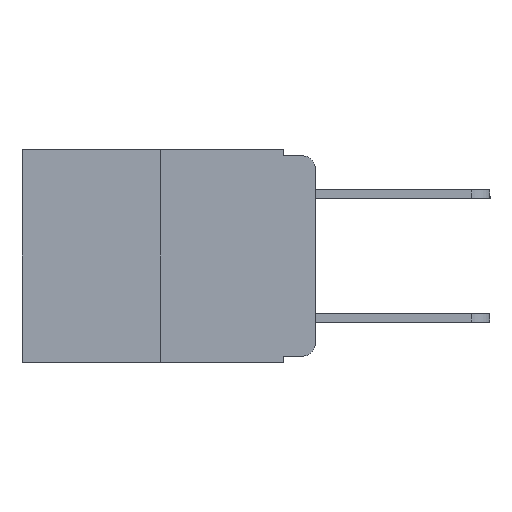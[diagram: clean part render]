
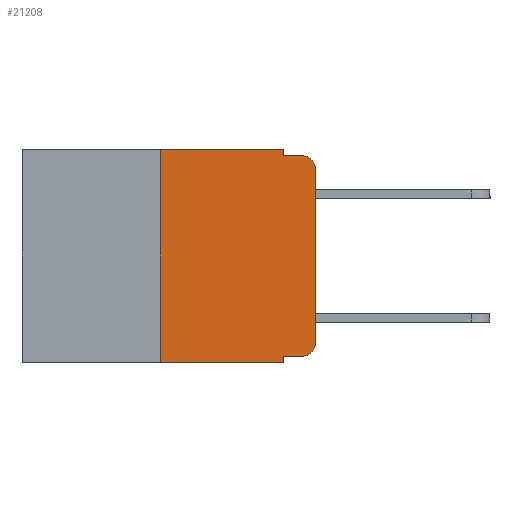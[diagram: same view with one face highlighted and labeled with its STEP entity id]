
A CAD part, left-side view. The second image highlights one B-rep face of the part: STEP entity #21208.
In plain terms, the highlighted planar face has unit normal (-1, 0, 0).
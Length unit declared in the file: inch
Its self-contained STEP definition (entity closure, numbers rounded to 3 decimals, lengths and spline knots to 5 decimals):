
#51 = CARTESIAN_POINT ( 'NONE',  ( 0., 0.02, -0.313 ) ) ;
#83 = EDGE_CURVE ( 'NONE', #9245, #9183, #15572, .T. ) ;
#554 = CARTESIAN_POINT ( 'NONE',  ( 0., 0.051, -0.333 ) ) ;
#600 = DIRECTION ( 'NONE',  ( 0., 0., 1. ) ) ;
#913 = ORIENTED_EDGE ( 'NONE', *, *, #4622, .F. ) ;
#1017 = LINE ( 'NONE', #14153, #20824 ) ;
#1240 = VERTEX_POINT ( 'NONE', #5856 ) ;
#1320 = VERTEX_POINT ( 'NONE', #21580 ) ;
#2061 = CIRCLE ( 'NONE', #3714, 0.02 ) ;
#2168 = DIRECTION ( 'NONE',  ( 0., 0., -1. ) ) ;
#2341 = LINE ( 'NONE', #16181, #12532 ) ;
#2483 = LINE ( 'NONE', #6446, #23901 ) ;
#2834 = ORIENTED_EDGE ( 'NONE', *, *, #15493, .F. ) ;
#3430 = DIRECTION ( 'NONE',  ( 0., -1., 0. ) ) ;
#3714 = AXIS2_PLACEMENT_3D ( 'NONE', #6079, #19696, #8152 ) ;
#4098 = DIRECTION ( 'NONE',  ( 0., -1., 0. ) ) ;
#4256 = EDGE_CURVE ( 'NONE', #25436, #9921, #2483, .T. ) ;
#4296 = VERTEX_POINT ( 'NONE', #20111 ) ;
#4622 = EDGE_CURVE ( 'NONE', #9921, #1320, #14458, .T. ) ;
#4873 = PLANE ( 'NONE',  #13325 ) ;
#4966 = VECTOR ( 'NONE', #13163, 39.37008 ) ;
#5633 = ORIENTED_EDGE ( 'NONE', *, *, #23953, .F. ) ;
#5644 = CARTESIAN_POINT ( 'NONE',  ( 0., 0.25, 0. ) ) ;
#5856 = CARTESIAN_POINT ( 'NONE',  ( 0., 0.02, -0.333 ) ) ;
#6028 = EDGE_CURVE ( 'NONE', #10557, #1320, #2061, .T. ) ;
#6079 = CARTESIAN_POINT ( 'NONE',  ( 0., 0.02, -0.03 ) ) ;
#6114 = CARTESIAN_POINT ( 'NONE',  ( 0., 0., -0.03 ) ) ;
#6156 = LINE ( 'NONE', #15862, #21080 ) ;
#6446 = CARTESIAN_POINT ( 'NONE',  ( 0., 0.051, 0. ) ) ;
#6512 = ORIENTED_EDGE ( 'NONE', *, *, #7581, .T. ) ;
#6797 = CARTESIAN_POINT ( 'NONE',  ( 0., 0., 0. ) ) ;
#6990 = DIRECTION ( 'NONE',  ( 0., 0., -1. ) ) ;
#7069 = CARTESIAN_POINT ( 'NONE',  ( 0., 0.25, 0. ) ) ;
#7581 = EDGE_CURVE ( 'NONE', #25396, #1240, #13008, .T. ) ;
#7684 = VECTOR ( 'NONE', #8191, 39.37008 ) ;
#8152 = DIRECTION ( 'NONE',  ( 0., 0., -1. ) ) ;
#8191 = DIRECTION ( 'NONE',  ( 0., -1., 0. ) ) ;
#9183 = VERTEX_POINT ( 'NONE', #7069 ) ;
#9184 = CARTESIAN_POINT ( 'NONE',  ( 0., 0.051, -0.343 ) ) ;
#9245 = VERTEX_POINT ( 'NONE', #24388 ) ;
#9268 = VECTOR ( 'NONE', #3430, 39.37008 ) ;
#9921 = VERTEX_POINT ( 'NONE', #25437 ) ;
#10101 = DIRECTION ( 'NONE',  ( 0., 0., -1. ) ) ;
#10139 = EDGE_CURVE ( 'NONE', #4296, #10557, #24393, .T. ) ;
#10557 = VERTEX_POINT ( 'NONE', #6114 ) ;
#11294 = FACE_OUTER_BOUND ( 'NONE', #24954, .T. ) ;
#12532 = VECTOR ( 'NONE', #21854, 39.37008 ) ;
#13008 = LINE ( 'NONE', #17864, #7684 ) ;
#13163 = DIRECTION ( 'NONE',  ( 0., 0., 1. ) ) ;
#13325 = AXIS2_PLACEMENT_3D ( 'NONE', #24239, #18639, #6990 ) ;
#13399 = VERTEX_POINT ( 'NONE', #9184 ) ;
#13525 = CARTESIAN_POINT ( 'NONE',  ( 0., 0.051, -0.01 ) ) ;
#13689 = ORIENTED_EDGE ( 'NONE', *, *, #6028, .T. ) ;
#14153 = CARTESIAN_POINT ( 'NONE',  ( 0., 0.473, -0.343 ) ) ;
#14273 = DIRECTION ( 'NONE',  ( -1., 0., 0. ) ) ;
#14335 = ORIENTED_EDGE ( 'NONE', *, *, #83, .F. ) ;
#14358 = VECTOR ( 'NONE', #600, 39.37008 ) ;
#14458 = LINE ( 'NONE', #13525, #9268 ) ;
#14669 = ORIENTED_EDGE ( 'NONE', *, *, #21024, .T. ) ;
#14813 = CARTESIAN_POINT ( 'NONE',  ( 0., 0.051, 0. ) ) ;
#15493 = EDGE_CURVE ( 'NONE', #25396, #13399, #6156, .T. ) ;
#15535 = CIRCLE ( 'NONE', #16319, 0.02 ) ;
#15572 = LINE ( 'NONE', #5644, #4966 ) ;
#15862 = CARTESIAN_POINT ( 'NONE',  ( 0., 0.051, 0. ) ) ;
#16181 = CARTESIAN_POINT ( 'NONE',  ( 0., 0.473, 0. ) ) ;
#16319 = AXIS2_PLACEMENT_3D ( 'NONE', #51, #14273, #2168 ) ;
#17864 = CARTESIAN_POINT ( 'NONE',  ( 0., 0.051, -0.333 ) ) ;
#18151 = DIRECTION ( 'NONE',  ( 0., 0., -1. ) ) ;
#18196 = ORIENTED_EDGE ( 'NONE', *, *, #10139, .T. ) ;
#18639 = DIRECTION ( 'NONE',  ( 1., 0., 0. ) ) ;
#19430 = ORIENTED_EDGE ( 'NONE', *, *, #4256, .F. ) ;
#19696 = DIRECTION ( 'NONE',  ( -1., 0., 0. ) ) ;
#20111 = CARTESIAN_POINT ( 'NONE',  ( 0., 0., -0.313 ) ) ;
#20824 = VECTOR ( 'NONE', #4098, 39.37008 ) ;
#21024 = EDGE_CURVE ( 'NONE', #1240, #4296, #15535, .T. ) ;
#21080 = VECTOR ( 'NONE', #10101, 39.37008 ) ;
#21208 = ADVANCED_FACE ( 'NONE', ( #11294 ), #4873, .F. ) ;
#21322 = ORIENTED_EDGE ( 'NONE', *, *, #25197, .T. ) ;
#21580 = CARTESIAN_POINT ( 'NONE',  ( 0., 0.02, -0.01 ) ) ;
#21854 = DIRECTION ( 'NONE',  ( 0., -1., 0. ) ) ;
#23901 = VECTOR ( 'NONE', #18151, 39.37008 ) ;
#23953 = EDGE_CURVE ( 'NONE', #9183, #25436, #2341, .T. ) ;
#24239 = CARTESIAN_POINT ( 'NONE',  ( 0., 0.473, 0. ) ) ;
#24388 = CARTESIAN_POINT ( 'NONE',  ( 0., 0.25, -0.343 ) ) ;
#24393 = LINE ( 'NONE', #6797, #14358 ) ;
#24954 = EDGE_LOOP ( 'NONE', ( #18196, #13689, #913, #19430, #5633, #14335, #21322, #2834, #6512, #14669 ) ) ;
#25197 = EDGE_CURVE ( 'NONE', #9245, #13399, #1017, .T. ) ;
#25396 = VERTEX_POINT ( 'NONE', #554 ) ;
#25436 = VERTEX_POINT ( 'NONE', #14813 ) ;
#25437 = CARTESIAN_POINT ( 'NONE',  ( 0., 0.051, -0.01 ) ) ;
